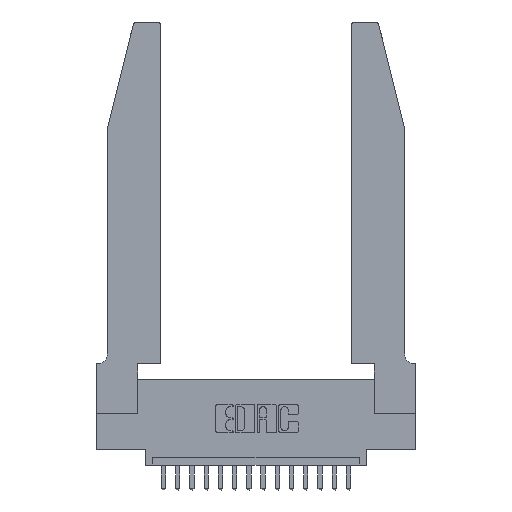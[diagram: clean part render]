
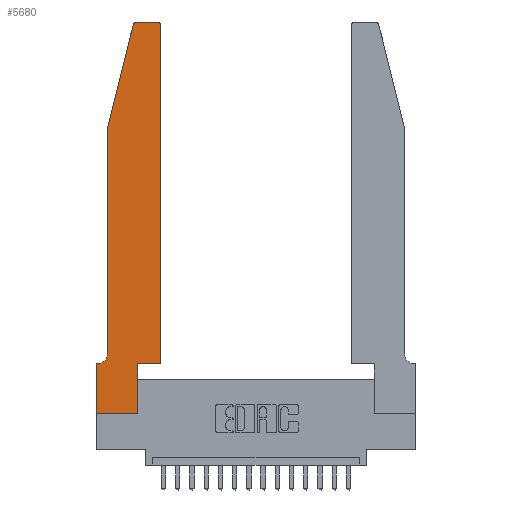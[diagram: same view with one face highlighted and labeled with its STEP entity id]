
A CAD part, top view. The second image highlights one B-rep face of the part: STEP entity #5680.
In plain terms, the highlighted planar face has unit normal (0, 0, 1).
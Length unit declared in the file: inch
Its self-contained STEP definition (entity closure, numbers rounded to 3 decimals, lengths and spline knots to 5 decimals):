
#153 = LINE ( 'NONE', #8335, #2956 ) ;
#222 = CARTESIAN_POINT ( 'NONE',  ( 0.0755, 0.35, 0.37 ) ) ;
#598 = CARTESIAN_POINT ( 'NONE',  ( 0., 0., 0.37 ) ) ;
#651 = CARTESIAN_POINT ( 'NONE',  ( 0.25487, 2.72718, 0.37 ) ) ;
#734 = CARTESIAN_POINT ( 'NONE',  ( 0.4505, 0.35, 0.37 ) ) ;
#787 = EDGE_CURVE ( 'NONE', #10604, #12990, #4477, .T. ) ;
#1782 = EDGE_CURVE ( 'NONE', #11192, #12507, #13505, .T. ) ;
#1811 = DIRECTION ( 'NONE',  ( 1., 0., 0. ) ) ;
#1864 = CARTESIAN_POINT ( 'NONE',  ( 0.0055, 0.35, 0.37 ) ) ;
#2079 = PLANE ( 'NONE',  #8353 ) ;
#2095 = EDGE_CURVE ( 'NONE', #16313, #7410, #16100, .T. ) ;
#2361 = DIRECTION ( 'NONE',  ( 0., 0., 1. ) ) ;
#2956 = VECTOR ( 'NONE', #7268, 39.37008 ) ;
#3035 = LINE ( 'NONE', #7149, #15807 ) ;
#3094 = CARTESIAN_POINT ( 'NONE',  ( 0.2865, 0., 0.37 ) ) ;
#3133 = CARTESIAN_POINT ( 'NONE',  ( 0.4505, 2.72, 0.37 ) ) ;
#3402 = ORIENTED_EDGE ( 'NONE', *, *, #12639, .T. ) ;
#3500 = VERTEX_POINT ( 'NONE', #7889 ) ;
#3505 = CARTESIAN_POINT ( 'NONE',  ( 0., 0., 0.37 ) ) ;
#3548 = ORIENTED_EDGE ( 'NONE', *, *, #19035, .T. ) ;
#3711 = LINE ( 'NONE', #9501, #7811 ) ;
#3967 = ORIENTED_EDGE ( 'NONE', *, *, #11494, .T. ) ;
#4021 = DIRECTION ( 'NONE',  ( 1., 0., 0. ) ) ;
#4132 = EDGE_CURVE ( 'NONE', #3500, #9301, #3035, .T. ) ;
#4173 = VECTOR ( 'NONE', #9025, 39.37008 ) ;
#4344 = CARTESIAN_POINT ( 'NONE',  ( 0.0055, 0.42, 0.37 ) ) ;
#4390 = LINE ( 'NONE', #222, #4173 ) ;
#4477 = LINE ( 'NONE', #18213, #15896 ) ;
#4776 = VERTEX_POINT ( 'NONE', #7167 ) ;
#5028 = ORIENTED_EDGE ( 'NONE', *, *, #13118, .T. ) ;
#5135 = CARTESIAN_POINT ( 'NONE',  ( 0., 0.35, 0.37 ) ) ;
#5340 = VERTEX_POINT ( 'NONE', #3133 ) ;
#5395 = LINE ( 'NONE', #3505, #12373 ) ;
#5431 = DIRECTION ( 'NONE',  ( 0., -1., 0. ) ) ;
#5564 = ORIENTED_EDGE ( 'NONE', *, *, #787, .T. ) ;
#5680 = ADVANCED_FACE ( 'NONE', ( #13550 ), #2079, .T. ) ;
#5825 = DIRECTION ( 'NONE',  ( 0., 0., -1. ) ) ;
#5886 = VERTEX_POINT ( 'NONE', #1864 ) ;
#6547 = LINE ( 'NONE', #734, #7265 ) ;
#7149 = CARTESIAN_POINT ( 'NONE',  ( 0.4505, 0.35, 0.37 ) ) ;
#7167 = CARTESIAN_POINT ( 'NONE',  ( 0., 0.35, 0.37 ) ) ;
#7265 = VECTOR ( 'NONE', #10606, 39.37008 ) ;
#7268 = DIRECTION ( 'NONE',  ( 0., 1., 0. ) ) ;
#7329 = AXIS2_PLACEMENT_3D ( 'NONE', #12643, #8137, #9618 ) ;
#7410 = VERTEX_POINT ( 'NONE', #10685 ) ;
#7811 = VECTOR ( 'NONE', #12479, 39.37008 ) ;
#7889 = CARTESIAN_POINT ( 'NONE',  ( 0.2865, 0.35, 0.37 ) ) ;
#8137 = DIRECTION ( 'NONE',  ( 0., 0., 1. ) ) ;
#8212 = DIRECTION ( 'NONE',  ( 0., 0., 1. ) ) ;
#8263 = EDGE_CURVE ( 'NONE', #8450, #16313, #3711, .T. ) ;
#8335 = CARTESIAN_POINT ( 'NONE',  ( 0.2865, 0.35, 0.37 ) ) ;
#8353 = AXIS2_PLACEMENT_3D ( 'NONE', #5135, #8212, #16957 ) ;
#8449 = CARTESIAN_POINT ( 'NONE',  ( 0.0755, 2., 0.37 ) ) ;
#8450 = VERTEX_POINT ( 'NONE', #651 ) ;
#8638 = EDGE_CURVE ( 'NONE', #12507, #8450, #17715, .T. ) ;
#8744 = ORIENTED_EDGE ( 'NONE', *, *, #11693, .T. ) ;
#9025 = DIRECTION ( 'NONE',  ( -1., 0., 0. ) ) ;
#9301 = VERTEX_POINT ( 'NONE', #11849 ) ;
#9501 = CARTESIAN_POINT ( 'NONE',  ( 0.0755, 2., 0.37 ) ) ;
#9618 = DIRECTION ( 'NONE',  ( 1., 0., 0. ) ) ;
#9647 = CIRCLE ( 'NONE', #11268, 0.07 ) ;
#10270 = VECTOR ( 'NONE', #19190, 39.37008 ) ;
#10411 = ORIENTED_EDGE ( 'NONE', *, *, #13694, .T. ) ;
#10604 = VERTEX_POINT ( 'NONE', #598 ) ;
#10606 = DIRECTION ( 'NONE',  ( 0., 1., 0. ) ) ;
#10685 = CARTESIAN_POINT ( 'NONE',  ( 0.0755, 0.42, 0.37 ) ) ;
#11192 = VERTEX_POINT ( 'NONE', #15435 ) ;
#11268 = AXIS2_PLACEMENT_3D ( 'NONE', #4344, #5825, #14754 ) ;
#11455 = ORIENTED_EDGE ( 'NONE', *, *, #8638, .T. ) ;
#11494 = EDGE_CURVE ( 'NONE', #12990, #3500, #153, .T. ) ;
#11664 = VECTOR ( 'NONE', #15605, 39.37008 ) ;
#11693 = EDGE_CURVE ( 'NONE', #7410, #5886, #9647, .T. ) ;
#11849 = CARTESIAN_POINT ( 'NONE',  ( 0.4505, 0.35, 0.37 ) ) ;
#12373 = VECTOR ( 'NONE', #5431, 39.37008 ) ;
#12459 = CARTESIAN_POINT ( 'NONE',  ( 0.0755, 2., 0.37 ) ) ;
#12479 = DIRECTION ( 'NONE',  ( -0.239, -0.971, 0. ) ) ;
#12507 = VERTEX_POINT ( 'NONE', #16351 ) ;
#12639 = EDGE_CURVE ( 'NONE', #9301, #5340, #6547, .T. ) ;
#12643 = CARTESIAN_POINT ( 'NONE',  ( 0.284, 2.72, 0.37 ) ) ;
#12824 = CARTESIAN_POINT ( 'NONE',  ( 0.4205, 2.72, 0.37 ) ) ;
#12990 = VERTEX_POINT ( 'NONE', #3094 ) ;
#13021 = ORIENTED_EDGE ( 'NONE', *, *, #2095, .T. ) ;
#13118 = EDGE_CURVE ( 'NONE', #4776, #10604, #5395, .T. ) ;
#13505 = LINE ( 'NONE', #17489, #10270 ) ;
#13550 = FACE_OUTER_BOUND ( 'NONE', #16081, .T. ) ;
#13694 = EDGE_CURVE ( 'NONE', #5340, #11192, #15523, .T. ) ;
#14459 = DIRECTION ( 'NONE',  ( 1., 0., 0. ) ) ;
#14754 = DIRECTION ( 'NONE',  ( -1., 0., 0. ) ) ;
#15435 = CARTESIAN_POINT ( 'NONE',  ( 0.4205, 2.75, 0.37 ) ) ;
#15523 = CIRCLE ( 'NONE', #15641, 0.03 ) ;
#15605 = DIRECTION ( 'NONE',  ( 0., -1., 0. ) ) ;
#15641 = AXIS2_PLACEMENT_3D ( 'NONE', #12824, #2361, #4021 ) ;
#15649 = ORIENTED_EDGE ( 'NONE', *, *, #4132, .T. ) ;
#15807 = VECTOR ( 'NONE', #14459, 39.37008 ) ;
#15896 = VECTOR ( 'NONE', #1811, 39.37008 ) ;
#16081 = EDGE_LOOP ( 'NONE', ( #16733, #11455, #18105, #13021, #8744, #3548, #5028, #5564, #3967, #15649, #3402, #10411 ) ) ;
#16100 = LINE ( 'NONE', #12459, #11664 ) ;
#16313 = VERTEX_POINT ( 'NONE', #8449 ) ;
#16351 = CARTESIAN_POINT ( 'NONE',  ( 0.284, 2.75, 0.37 ) ) ;
#16733 = ORIENTED_EDGE ( 'NONE', *, *, #1782, .T. ) ;
#16957 = DIRECTION ( 'NONE',  ( 1., 0., 0. ) ) ;
#17489 = CARTESIAN_POINT ( 'NONE',  ( 0.2605, 2.75, 0.37 ) ) ;
#17715 = CIRCLE ( 'NONE', #7329, 0.03 ) ;
#18105 = ORIENTED_EDGE ( 'NONE', *, *, #8263, .T. ) ;
#18213 = CARTESIAN_POINT ( 'NONE',  ( 0., 0., 0.37 ) ) ;
#19035 = EDGE_CURVE ( 'NONE', #5886, #4776, #4390, .T. ) ;
#19190 = DIRECTION ( 'NONE',  ( -1., 0., 0. ) ) ;
